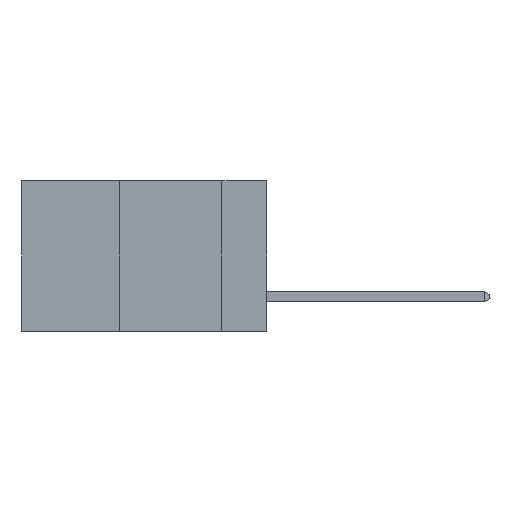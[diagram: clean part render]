
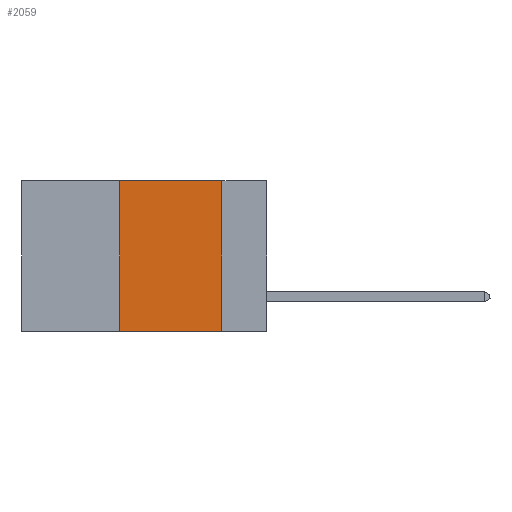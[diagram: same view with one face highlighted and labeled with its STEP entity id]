
A CAD part, left-side view. The second image highlights one B-rep face of the part: STEP entity #2059.
In plain terms, the highlighted planar face has unit normal (-1, 0, 0).
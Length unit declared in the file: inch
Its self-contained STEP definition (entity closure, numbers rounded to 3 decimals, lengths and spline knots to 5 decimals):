
#13 = PLANE ( 'NONE',  #7073 ) ;
#108 = VECTOR ( 'NONE', #7573, 39.37008 ) ;
#1531 = CARTESIAN_POINT ( 'NONE',  ( 0., 0.6, 0. ) ) ;
#1541 = LINE ( 'NONE', #15736, #18415 ) ;
#2059 = ADVANCED_FACE ( 'NONE', ( #12708 ), #13, .F. ) ;
#2151 = ORIENTED_EDGE ( 'NONE', *, *, #5082, .F. ) ;
#2893 = VERTEX_POINT ( 'NONE', #15363 ) ;
#3413 = EDGE_CURVE ( 'NONE', #13006, #17373, #19176, .T. ) ;
#4081 = CARTESIAN_POINT ( 'NONE',  ( 0., 0.6, -0.37 ) ) ;
#4286 = ORIENTED_EDGE ( 'NONE', *, *, #7736, .F. ) ;
#5082 = EDGE_CURVE ( 'NONE', #12683, #2893, #6243, .T. ) ;
#5937 = CARTESIAN_POINT ( 'NONE',  ( 0., 0.36, 0. ) ) ;
#6243 = LINE ( 'NONE', #5937, #108 ) ;
#6481 = DIRECTION ( 'NONE',  ( 0., -1., 0. ) ) ;
#7073 = AXIS2_PLACEMENT_3D ( 'NONE', #1531, #11960, #17924 ) ;
#7573 = DIRECTION ( 'NONE',  ( 0., 0., 1. ) ) ;
#7736 = EDGE_CURVE ( 'NONE', #2893, #13006, #1541, .T. ) ;
#8299 = EDGE_CURVE ( 'NONE', #12683, #17373, #12096, .T. ) ;
#11033 = DIRECTION ( 'NONE',  ( 0., 0., -1. ) ) ;
#11716 = VECTOR ( 'NONE', #11033, 39.37008 ) ;
#11960 = DIRECTION ( 'NONE',  ( 1., 0., 0. ) ) ;
#12096 = LINE ( 'NONE', #4081, #16556 ) ;
#12683 = VERTEX_POINT ( 'NONE', #16786 ) ;
#12708 = FACE_OUTER_BOUND ( 'NONE', #17283, .T. ) ;
#12799 = ORIENTED_EDGE ( 'NONE', *, *, #3413, .F. ) ;
#13006 = VERTEX_POINT ( 'NONE', #19300 ) ;
#14711 = CARTESIAN_POINT ( 'NONE',  ( 0., 0.11, 0. ) ) ;
#15363 = CARTESIAN_POINT ( 'NONE',  ( 0., 0.36, 0. ) ) ;
#15392 = CARTESIAN_POINT ( 'NONE',  ( 0., 0.11, -0.37 ) ) ;
#15736 = CARTESIAN_POINT ( 'NONE',  ( 0., 0.6, 0. ) ) ;
#16238 = ORIENTED_EDGE ( 'NONE', *, *, #8299, .T. ) ;
#16556 = VECTOR ( 'NONE', #19242, 39.37008 ) ;
#16786 = CARTESIAN_POINT ( 'NONE',  ( 0., 0.36, -0.37 ) ) ;
#17283 = EDGE_LOOP ( 'NONE', ( #12799, #4286, #2151, #16238 ) ) ;
#17373 = VERTEX_POINT ( 'NONE', #15392 ) ;
#17924 = DIRECTION ( 'NONE',  ( 0., 0., -1. ) ) ;
#18415 = VECTOR ( 'NONE', #6481, 39.37008 ) ;
#19176 = LINE ( 'NONE', #14711, #11716 ) ;
#19242 = DIRECTION ( 'NONE',  ( 0., -1., 0. ) ) ;
#19300 = CARTESIAN_POINT ( 'NONE',  ( 0., 0.11, 0. ) ) ;
